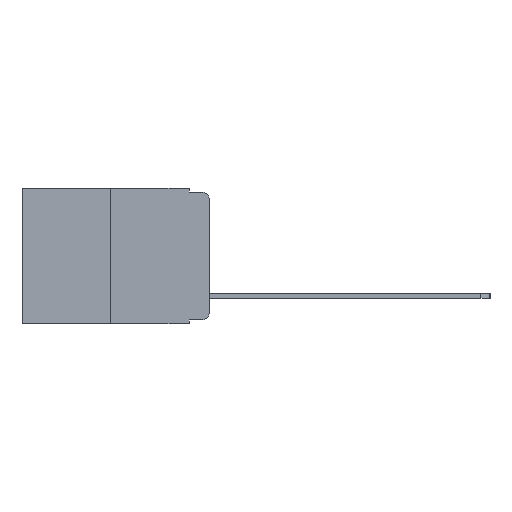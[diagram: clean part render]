
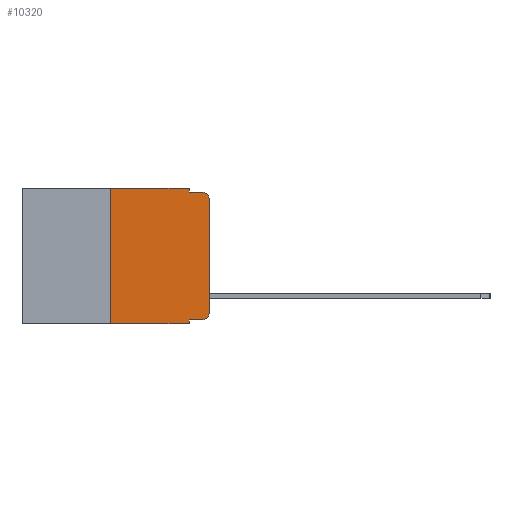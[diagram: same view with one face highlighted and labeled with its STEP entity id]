
A CAD part, left-side view. The second image highlights one B-rep face of the part: STEP entity #10320.
In plain terms, the highlighted planar face has unit normal (-1, 0, 0).
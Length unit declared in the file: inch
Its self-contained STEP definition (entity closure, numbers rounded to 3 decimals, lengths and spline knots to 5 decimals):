
#76 = ORIENTED_EDGE ( 'NONE', *, *, #2409, .F. ) ;
#87 = ORIENTED_EDGE ( 'NONE', *, *, #5383, .F. ) ;
#145 = DIRECTION ( 'NONE',  ( 0., 0., 1. ) ) ;
#163 = CARTESIAN_POINT ( 'NONE',  ( 0., 0.02, -0.333 ) ) ;
#336 = VECTOR ( 'NONE', #7138, 39.37008 ) ;
#387 = ORIENTED_EDGE ( 'NONE', *, *, #2441, .F. ) ;
#397 = CARTESIAN_POINT ( 'NONE',  ( 0., 0.02, -0.01 ) ) ;
#404 = ORIENTED_EDGE ( 'NONE', *, *, #5474, .T. ) ;
#483 = VECTOR ( 'NONE', #4421, 39.37008 ) ;
#665 = ORIENTED_EDGE ( 'NONE', *, *, #2476, .F. ) ;
#844 = ORIENTED_EDGE ( 'NONE', *, *, #2528, .T. ) ;
#881 = ORIENTED_EDGE ( 'NONE', *, *, #2550, .T. ) ;
#1202 = CARTESIAN_POINT ( 'NONE',  ( 0., 0.25, 0. ) ) ;
#1572 = LINE ( 'NONE', #6550, #8406 ) ;
#1659 = DIRECTION ( 'NONE',  ( 0., 0., -1. ) ) ;
#1790 = EDGE_CURVE ( 'NONE', #11382, #9482, #5839, .T. ) ;
#1965 = AXIS2_PLACEMENT_3D ( 'NONE', #4454, #7032, #1659 ) ;
#2346 = EDGE_CURVE ( 'NONE', #3320, #9482, #7678, .T. ) ;
#2409 = EDGE_CURVE ( 'NONE', #11070, #3320, #4889, .T. ) ;
#2441 = EDGE_CURVE ( 'NONE', #5219, #3423, #8358, .T. ) ;
#2476 = EDGE_CURVE ( 'NONE', #3100, #5797, #8109, .T. ) ;
#2528 = EDGE_CURVE ( 'NONE', #3100, #10535, #5282, .T. ) ;
#2550 = EDGE_CURVE ( 'NONE', #10535, #3679, #9268, .T. ) ;
#2835 = DIRECTION ( 'NONE',  ( 0., 0., -1. ) ) ;
#3100 = VERTEX_POINT ( 'NONE', #4708 ) ;
#3320 = VERTEX_POINT ( 'NONE', #5119 ) ;
#3404 = FACE_OUTER_BOUND ( 'NONE', #8244, .T. ) ;
#3423 = VERTEX_POINT ( 'NONE', #9539 ) ;
#3432 = CARTESIAN_POINT ( 'NONE',  ( 0., 0.051, -0.343 ) ) ;
#3679 = VERTEX_POINT ( 'NONE', #10816 ) ;
#4010 = CARTESIAN_POINT ( 'NONE',  ( 0., 0.051, -0.01 ) ) ;
#4421 = DIRECTION ( 'NONE',  ( 0., -1., 0. ) ) ;
#4454 = CARTESIAN_POINT ( 'NONE',  ( 0., 0.473, 0. ) ) ;
#4708 = CARTESIAN_POINT ( 'NONE',  ( 0., 0.051, -0.333 ) ) ;
#4790 = VECTOR ( 'NONE', #4929, 39.37008 ) ;
#4849 = ORIENTED_EDGE ( 'NONE', *, *, #2346, .F. ) ;
#4889 = LINE ( 'NONE', #6081, #11318 ) ;
#4929 = DIRECTION ( 'NONE',  ( 0., -1., 0. ) ) ;
#5119 = CARTESIAN_POINT ( 'NONE',  ( 0., 0.051, -0.01 ) ) ;
#5201 = DIRECTION ( 'NONE',  ( -1., 0., 0. ) ) ;
#5219 = VERTEX_POINT ( 'NONE', #10476 ) ;
#5282 = LINE ( 'NONE', #8180, #336 ) ;
#5383 = EDGE_CURVE ( 'NONE', #3423, #11070, #1572, .T. ) ;
#5474 = EDGE_CURVE ( 'NONE', #5219, #5797, #7041, .T. ) ;
#5558 = VECTOR ( 'NONE', #2835, 39.37008 ) ;
#5797 = VERTEX_POINT ( 'NONE', #3432 ) ;
#5839 = CIRCLE ( 'NONE', #6215, 0.02 ) ;
#5910 = CARTESIAN_POINT ( 'NONE',  ( 0., 0.02, -0.313 ) ) ;
#5936 = DIRECTION ( 'NONE',  ( 0., 0., 1. ) ) ;
#6081 = CARTESIAN_POINT ( 'NONE',  ( 0., 0.051, 0. ) ) ;
#6180 = PLANE ( 'NONE',  #1965 ) ;
#6215 = AXIS2_PLACEMENT_3D ( 'NONE', #7130, #5201, #8384 ) ;
#6550 = CARTESIAN_POINT ( 'NONE',  ( 0., 0.473, 0. ) ) ;
#6866 = ORIENTED_EDGE ( 'NONE', *, *, #11291, .T. ) ;
#7032 = DIRECTION ( 'NONE',  ( 1., 0., 0. ) ) ;
#7041 = LINE ( 'NONE', #7443, #4790 ) ;
#7130 = CARTESIAN_POINT ( 'NONE',  ( 0., 0.02, -0.03 ) ) ;
#7138 = DIRECTION ( 'NONE',  ( 0., -1., 0. ) ) ;
#7368 = ORIENTED_EDGE ( 'NONE', *, *, #1790, .T. ) ;
#7443 = CARTESIAN_POINT ( 'NONE',  ( 0., 0.473, -0.343 ) ) ;
#7678 = LINE ( 'NONE', #4010, #483 ) ;
#8104 = CARTESIAN_POINT ( 'NONE',  ( 0., 0.051, 0. ) ) ;
#8107 = DIRECTION ( 'NONE',  ( 0., 0., -1. ) ) ;
#8109 = LINE ( 'NONE', #8243, #5558 ) ;
#8180 = CARTESIAN_POINT ( 'NONE',  ( 0., 0.051, -0.333 ) ) ;
#8243 = CARTESIAN_POINT ( 'NONE',  ( 0., 0.051, 0. ) ) ;
#8244 = EDGE_LOOP ( 'NONE', ( #6866, #7368, #4849, #76, #87, #387, #404, #665, #844, #881 ) ) ;
#8358 = LINE ( 'NONE', #1202, #8607 ) ;
#8384 = DIRECTION ( 'NONE',  ( 0., 0., -1. ) ) ;
#8406 = VECTOR ( 'NONE', #9127, 39.37008 ) ;
#8607 = VECTOR ( 'NONE', #145, 39.37008 ) ;
#8620 = CARTESIAN_POINT ( 'NONE',  ( 0., 0., -0.03 ) ) ;
#8903 = LINE ( 'NONE', #10974, #11343 ) ;
#8968 = DIRECTION ( 'NONE',  ( -1., 0., 0. ) ) ;
#9127 = DIRECTION ( 'NONE',  ( 0., -1., 0. ) ) ;
#9268 = CIRCLE ( 'NONE', #10222, 0.02 ) ;
#9482 = VERTEX_POINT ( 'NONE', #397 ) ;
#9539 = CARTESIAN_POINT ( 'NONE',  ( 0., 0.25, 0. ) ) ;
#9949 = DIRECTION ( 'NONE',  ( 0., 0., -1. ) ) ;
#10222 = AXIS2_PLACEMENT_3D ( 'NONE', #5910, #8968, #9949 ) ;
#10320 = ADVANCED_FACE ( 'NONE', ( #3404 ), #6180, .F. ) ;
#10476 = CARTESIAN_POINT ( 'NONE',  ( 0., 0.25, -0.343 ) ) ;
#10535 = VERTEX_POINT ( 'NONE', #163 ) ;
#10816 = CARTESIAN_POINT ( 'NONE',  ( 0., 0., -0.313 ) ) ;
#10974 = CARTESIAN_POINT ( 'NONE',  ( 0., 0., 0. ) ) ;
#11070 = VERTEX_POINT ( 'NONE', #8104 ) ;
#11291 = EDGE_CURVE ( 'NONE', #3679, #11382, #8903, .T. ) ;
#11318 = VECTOR ( 'NONE', #8107, 39.37008 ) ;
#11343 = VECTOR ( 'NONE', #5936, 39.37008 ) ;
#11382 = VERTEX_POINT ( 'NONE', #8620 ) ;
